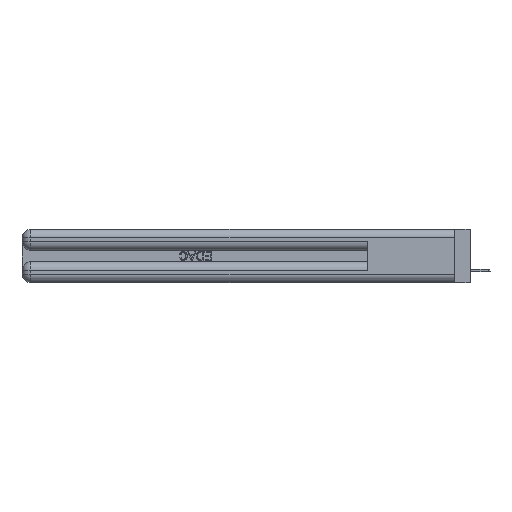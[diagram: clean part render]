
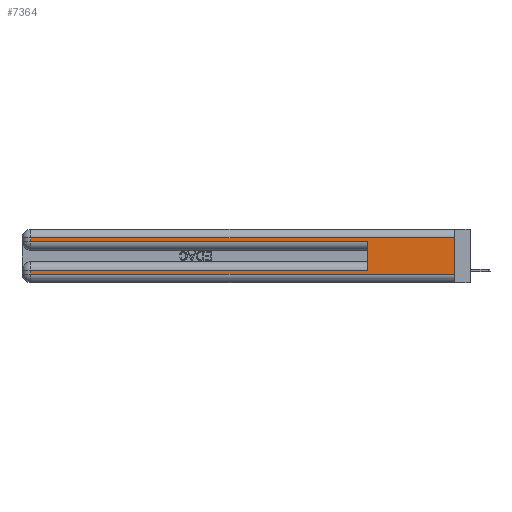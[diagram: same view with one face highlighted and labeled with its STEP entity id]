
A CAD part, left-side view. The second image highlights one B-rep face of the part: STEP entity #7364.
In plain terms, the highlighted planar face has unit normal (-1, 0, 0).
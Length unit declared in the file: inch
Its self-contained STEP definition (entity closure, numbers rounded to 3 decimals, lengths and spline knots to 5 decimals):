
#513 = CARTESIAN_POINT ( 'NONE',  ( 0., 0., 0.06 ) ) ;
#798 = CARTESIAN_POINT ( 'NONE',  ( 0., 2.94, 0.31 ) ) ;
#1403 = AXIS2_PLACEMENT_3D ( 'NONE', #15519, #15057, #32849 ) ;
#1570 = VECTOR ( 'NONE', #11447, 39.37008 ) ;
#2297 = VERTEX_POINT ( 'NONE', #13310 ) ;
#3355 = CARTESIAN_POINT ( 'NONE',  ( 0., 0.6, 0.145 ) ) ;
#3427 = EDGE_CURVE ( 'NONE', #2297, #6573, #43325, .T. ) ;
#4045 = CARTESIAN_POINT ( 'NONE',  ( 0., 0.6, 0.085 ) ) ;
#4237 = VECTOR ( 'NONE', #41975, 39.37008 ) ;
#6351 = DIRECTION ( 'NONE',  ( 0., 1., 0. ) ) ;
#6573 = VERTEX_POINT ( 'NONE', #25658 ) ;
#6641 = VECTOR ( 'NONE', #27622, 39.37008 ) ;
#7364 = ADVANCED_FACE ( 'NONE', ( #43378 ), #8031, .F. ) ;
#7770 = VECTOR ( 'NONE', #13861, 39.37008 ) ;
#8031 = PLANE ( 'NONE',  #1403 ) ;
#9412 = VECTOR ( 'NONE', #36850, 39.37008 ) ;
#9427 = VECTOR ( 'NONE', #38765, 39.37008 ) ;
#10266 = VERTEX_POINT ( 'NONE', #31716 ) ;
#10344 = CARTESIAN_POINT ( 'NONE',  ( 0., 2.94, 0.37 ) ) ;
#10534 = EDGE_CURVE ( 'NONE', #10266, #22550, #39112, .T. ) ;
#11217 = LINE ( 'NONE', #11907, #1570 ) ;
#11447 = DIRECTION ( 'NONE',  ( 0., 0., -1. ) ) ;
#11708 = VECTOR ( 'NONE', #12912, 39.37008 ) ;
#11907 = CARTESIAN_POINT ( 'NONE',  ( 0., 2.94, 0.37 ) ) ;
#12320 = ORIENTED_EDGE ( 'NONE', *, *, #10534, .T. ) ;
#12912 = DIRECTION ( 'NONE',  ( 0., 0., -1. ) ) ;
#13206 = ORIENTED_EDGE ( 'NONE', *, *, #31614, .T. ) ;
#13310 = CARTESIAN_POINT ( 'NONE',  ( 0., 2.94, 0.085 ) ) ;
#13685 = ORIENTED_EDGE ( 'NONE', *, *, #3427, .T. ) ;
#13861 = DIRECTION ( 'NONE',  ( 0., 0., -1. ) ) ;
#14423 = LINE ( 'NONE', #28717, #9427 ) ;
#15057 = DIRECTION ( 'NONE',  ( 1., 0., 0. ) ) ;
#15488 = VERTEX_POINT ( 'NONE', #31802 ) ;
#15519 = CARTESIAN_POINT ( 'NONE',  ( 0., 0., 0.37 ) ) ;
#16942 = EDGE_CURVE ( 'NONE', #6573, #44520, #14423, .T. ) ;
#17494 = EDGE_CURVE ( 'NONE', #10266, #44520, #44524, .T. ) ;
#18309 = VERTEX_POINT ( 'NONE', #27059 ) ;
#19709 = CARTESIAN_POINT ( 'NONE',  ( 0., 0., 0.37 ) ) ;
#19808 = EDGE_LOOP ( 'NONE', ( #33587, #12320, #40585, #43631, #35577, #13206, #13685, #23612 ) ) ;
#20261 = VERTEX_POINT ( 'NONE', #4045 ) ;
#22550 = VERTEX_POINT ( 'NONE', #798 ) ;
#22588 = CARTESIAN_POINT ( 'NONE',  ( 0., 0., 0.085 ) ) ;
#23612 = ORIENTED_EDGE ( 'NONE', *, *, #16942, .T. ) ;
#25658 = CARTESIAN_POINT ( 'NONE',  ( 0., 2.94, 0.06 ) ) ;
#27059 = CARTESIAN_POINT ( 'NONE',  ( 0., 2.94, 0.285 ) ) ;
#27394 = CARTESIAN_POINT ( 'NONE',  ( 0., 0., 0.285 ) ) ;
#27622 = DIRECTION ( 'NONE',  ( 0., -1., 0. ) ) ;
#28717 = CARTESIAN_POINT ( 'NONE',  ( 0., 0., 0.06 ) ) ;
#29623 = LINE ( 'NONE', #22588, #9412 ) ;
#31614 = EDGE_CURVE ( 'NONE', #20261, #2297, #29623, .T. ) ;
#31716 = CARTESIAN_POINT ( 'NONE',  ( 0., 0., 0.31 ) ) ;
#31802 = CARTESIAN_POINT ( 'NONE',  ( 0., 0.6, 0.285 ) ) ;
#31899 = EDGE_CURVE ( 'NONE', #20261, #15488, #38474, .T. ) ;
#32849 = DIRECTION ( 'NONE',  ( 0., 0., -1. ) ) ;
#33587 = ORIENTED_EDGE ( 'NONE', *, *, #17494, .F. ) ;
#34936 = EDGE_CURVE ( 'NONE', #18309, #15488, #41660, .T. ) ;
#35577 = ORIENTED_EDGE ( 'NONE', *, *, #31899, .F. ) ;
#36850 = DIRECTION ( 'NONE',  ( 0., 1., 0. ) ) ;
#37491 = VECTOR ( 'NONE', #6351, 39.37008 ) ;
#38474 = LINE ( 'NONE', #3355, #4237 ) ;
#38765 = DIRECTION ( 'NONE',  ( 0., -1., 0. ) ) ;
#39013 = EDGE_CURVE ( 'NONE', #22550, #18309, #11217, .T. ) ;
#39112 = LINE ( 'NONE', #41924, #37491 ) ;
#40585 = ORIENTED_EDGE ( 'NONE', *, *, #39013, .T. ) ;
#41660 = LINE ( 'NONE', #27394, #6641 ) ;
#41924 = CARTESIAN_POINT ( 'NONE',  ( 0., 0., 0.31 ) ) ;
#41975 = DIRECTION ( 'NONE',  ( 0., 0., 1. ) ) ;
#43325 = LINE ( 'NONE', #10344, #7770 ) ;
#43378 = FACE_OUTER_BOUND ( 'NONE', #19808, .T. ) ;
#43631 = ORIENTED_EDGE ( 'NONE', *, *, #34936, .T. ) ;
#44520 = VERTEX_POINT ( 'NONE', #513 ) ;
#44524 = LINE ( 'NONE', #19709, #11708 ) ;
